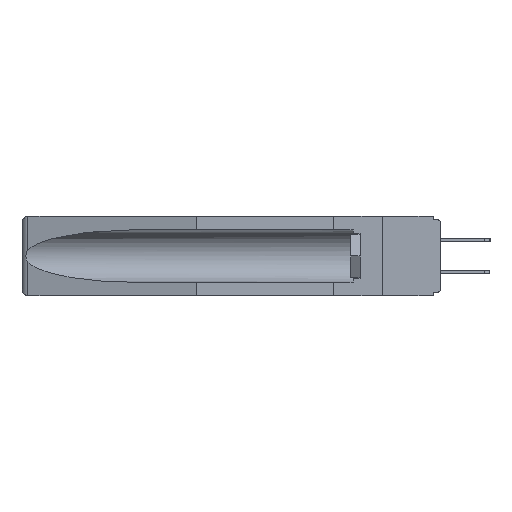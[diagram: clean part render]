
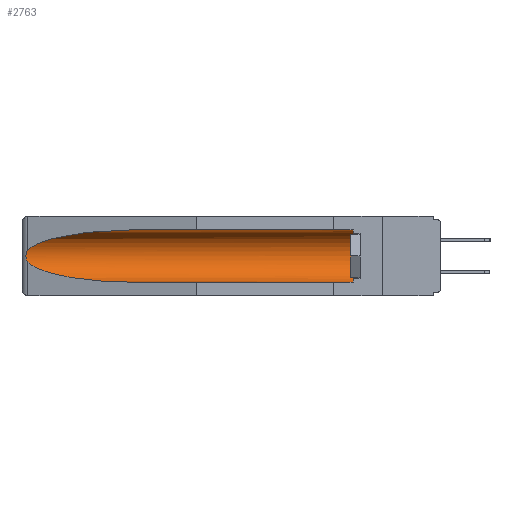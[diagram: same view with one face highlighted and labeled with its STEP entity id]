
A CAD part, left-side view. The second image highlights one B-rep face of the part: STEP entity #2763.
In plain terms, the highlighted cylindrical face has radius 2.857 mm (diameter 5.715 mm), a partial arc.
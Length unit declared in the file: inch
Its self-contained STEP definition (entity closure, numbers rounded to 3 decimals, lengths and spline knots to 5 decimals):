
#589 = CARTESIAN_POINT ( 'NONE',  ( 0.26537, 1.52718, -0.19328 ) ) ;
#1087 = ORIENTED_EDGE ( 'NONE', *, *, #8848, .T. ) ;
#1111 = VERTEX_POINT ( 'NONE', #18005 ) ;
#1580 =( BOUNDED_CURVE ( )  B_SPLINE_CURVE ( 3, ( #11833, #20774, #12983, #20694 ),
 .UNSPECIFIED., .F., .F. ) 
 B_SPLINE_CURVE_WITH_KNOTS ( ( 4, 4 ),
 ( 0.1948, 1.5708 ),
 .UNSPECIFIED. ) 
 CURVE ( )  GEOMETRIC_REPRESENTATION_ITEM ( )  RATIONAL_B_SPLINE_CURVE ( ( 1., 0.848, 0.848, 1. ) ) 
 REPRESENTATION_ITEM ( '' )  );
#2067 = CARTESIAN_POINT ( 'NONE',  ( 0.25451, 1.48313, -0.09465 ) ) ;
#2313 =( BOUNDED_CURVE ( )  B_SPLINE_CURVE ( 3, ( #5533, #7627, #2067, #20976 ),
 .UNSPECIFIED., .F., .F. ) 
 B_SPLINE_CURVE_WITH_KNOTS ( ( 4, 4 ),
 ( 4.71239, 6.08839 ),
 .UNSPECIFIED. ) 
 CURVE ( )  GEOMETRIC_REPRESENTATION_ITEM ( )  RATIONAL_B_SPLINE_CURVE ( ( 1., 0.848, 0.848, 1. ) ) 
 REPRESENTATION_ITEM ( '' )  );
#2763 = ADVANCED_FACE ( 'NONE', ( #5591 ), #24095, .F. ) ;
#2900 = CARTESIAN_POINT ( 'NONE',  ( 0.155, 0.126, -0.284 ) ) ;
#3097 = CARTESIAN_POINT ( 'NONE',  ( 0.26655, 1.53094, -0.18657 ) ) ;
#4000 = VERTEX_POINT ( 'NONE', #9565 ) ;
#4090 = EDGE_CURVE ( 'NONE', #1111, #13342, #1580, .T. ) ;
#4182 = LINE ( 'NONE', #6629, #23902 ) ;
#4875 = EDGE_LOOP ( 'NONE', ( #14780, #16845, #24032, #8323, #21314, #1087 ) ) ;
#4919 = CARTESIAN_POINT ( 'NONE',  ( 0.2673, 1.5327, -0.16383 ) ) ;
#5533 = CARTESIAN_POINT ( 'NONE',  ( 0.155, 1.07973, -0.059 ) ) ;
#5591 = FACE_OUTER_BOUND ( 'NONE', #4875, .T. ) ;
#5882 = DIRECTION ( 'NONE',  ( 0., 0., 1. ) ) ;
#6629 = CARTESIAN_POINT ( 'NONE',  ( 0.155, -0.30754, -0.284 ) ) ;
#6689 = CARTESIAN_POINT ( 'NONE',  ( 0.26537, 1.52718, -0.14972 ) ) ;
#6839 = CARTESIAN_POINT ( 'NONE',  ( 0.2675, 1.53308, -0.17534 ) ) ;
#6866 = DIRECTION ( 'NONE',  ( 0., 1., 0. ) ) ;
#7481 = DIRECTION ( 'NONE',  ( 0., 1., 0. ) ) ;
#7627 = CARTESIAN_POINT ( 'NONE',  ( 0.21114, 1.30732, -0.059 ) ) ;
#7954 = CARTESIAN_POINT ( 'NONE',  ( 0.155, 1.07973, -0.284 ) ) ;
#8236 = B_SPLINE_CURVE_WITH_KNOTS ( 'NONE', 3,
 ( #6689, #22031, #10585, #4919, #18356, #6839, #20179, #3097, #8739, #589 ),
 .UNSPECIFIED., .F., .F.,
 ( 4, 2, 2, 2, 4 ),
 ( 0., 0.00029, 0.00058, 0.00087, 0.00117 ),
 .UNSPECIFIED. ) ;
#8323 = ORIENTED_EDGE ( 'NONE', *, *, #11297, .F. ) ;
#8622 = CARTESIAN_POINT ( 'NONE',  ( 0.155, -0.30754, -0.059 ) ) ;
#8739 = CARTESIAN_POINT ( 'NONE',  ( 0.26597, 1.5296, -0.19026 ) ) ;
#8848 = EDGE_CURVE ( 'NONE', #4000, #17271, #13039, .T. ) ;
#9400 = DIRECTION ( 'NONE',  ( 0., 0., 1. ) ) ;
#9565 = CARTESIAN_POINT ( 'NONE',  ( 0.155, 0.126, -0.059 ) ) ;
#9705 = VECTOR ( 'NONE', #10400, 39.37008 ) ;
#10400 = DIRECTION ( 'NONE',  ( 0., 1., 0. ) ) ;
#10585 = CARTESIAN_POINT ( 'NONE',  ( 0.26654, 1.53092, -0.15636 ) ) ;
#11248 = CARTESIAN_POINT ( 'NONE',  ( 0.155, -0.30754, -0.1715 ) ) ;
#11297 = EDGE_CURVE ( 'NONE', #14835, #13342, #4182, .T. ) ;
#11600 = EDGE_CURVE ( 'NONE', #19167, #1111, #8236, .T. ) ;
#11833 = CARTESIAN_POINT ( 'NONE',  ( 0.26537, 1.52718, -0.19328 ) ) ;
#12983 = CARTESIAN_POINT ( 'NONE',  ( 0.21114, 1.30732, -0.284 ) ) ;
#13039 = LINE ( 'NONE', #8622, #9705 ) ;
#13342 = VERTEX_POINT ( 'NONE', #7954 ) ;
#13437 = DIRECTION ( 'NONE',  ( 0., -1., 0. ) ) ;
#14096 = AXIS2_PLACEMENT_3D ( 'NONE', #17342, #13437, #5882 ) ;
#14780 = ORIENTED_EDGE ( 'NONE', *, *, #20437, .T. ) ;
#14835 = VERTEX_POINT ( 'NONE', #2900 ) ;
#16845 = ORIENTED_EDGE ( 'NONE', *, *, #11600, .T. ) ;
#17271 = VERTEX_POINT ( 'NONE', #18811 ) ;
#17342 = CARTESIAN_POINT ( 'NONE',  ( 0.155, 0.126, -0.1715 ) ) ;
#18005 = CARTESIAN_POINT ( 'NONE',  ( 0.26537, 1.52718, -0.19328 ) ) ;
#18356 = CARTESIAN_POINT ( 'NONE',  ( 0.2675, 1.53308, -0.16763 ) ) ;
#18811 = CARTESIAN_POINT ( 'NONE',  ( 0.155, 1.07973, -0.059 ) ) ;
#18947 = CARTESIAN_POINT ( 'NONE',  ( 0.26537, 1.52718, -0.14972 ) ) ;
#19167 = VERTEX_POINT ( 'NONE', #18947 ) ;
#20179 = CARTESIAN_POINT ( 'NONE',  ( 0.2673, 1.53269, -0.17917 ) ) ;
#20437 = EDGE_CURVE ( 'NONE', #17271, #19167, #2313, .T. ) ;
#20632 = EDGE_CURVE ( 'NONE', #14835, #4000, #24451, .T. ) ;
#20694 = CARTESIAN_POINT ( 'NONE',  ( 0.155, 1.07973, -0.284 ) ) ;
#20774 = CARTESIAN_POINT ( 'NONE',  ( 0.25451, 1.48313, -0.24835 ) ) ;
#20976 = CARTESIAN_POINT ( 'NONE',  ( 0.26537, 1.52718, -0.14972 ) ) ;
#21314 = ORIENTED_EDGE ( 'NONE', *, *, #20632, .T. ) ;
#21811 = AXIS2_PLACEMENT_3D ( 'NONE', #11248, #7481, #9400 ) ;
#22031 = CARTESIAN_POINT ( 'NONE',  ( 0.26597, 1.52961, -0.15275 ) ) ;
#23902 = VECTOR ( 'NONE', #6866, 39.37008 ) ;
#24032 = ORIENTED_EDGE ( 'NONE', *, *, #4090, .T. ) ;
#24095 = CYLINDRICAL_SURFACE ( 'NONE', #21811, 0.1125 ) ;
#24451 = CIRCLE ( 'NONE', #14096, 0.1125 ) ;
